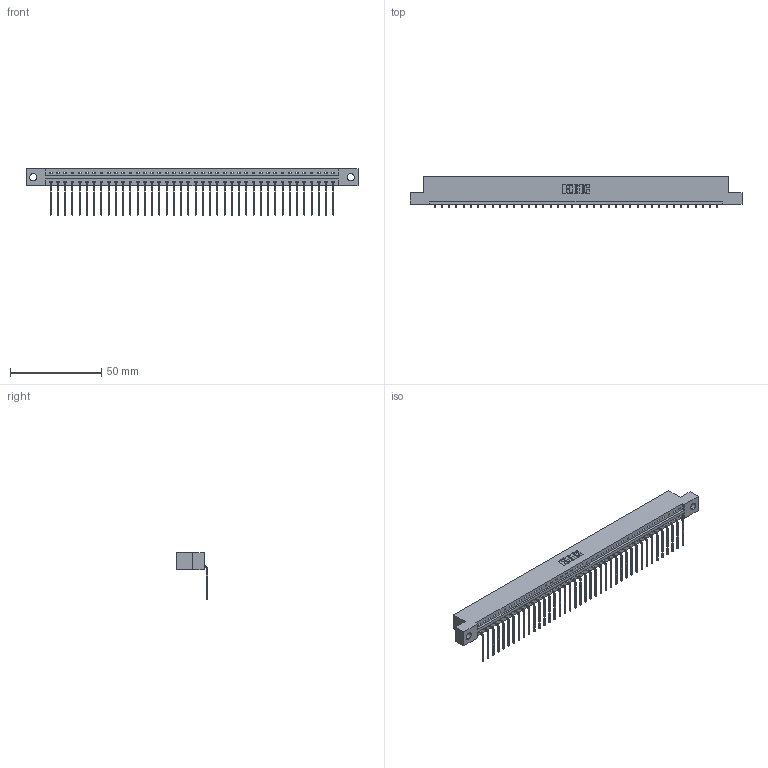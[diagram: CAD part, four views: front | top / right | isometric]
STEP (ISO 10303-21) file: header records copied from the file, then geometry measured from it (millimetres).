
FILE_DESCRIPTION (( 'STEP AP203' ), '1' );
FILE_NAME ('387-040-559-104.STEP', '2018-09-19T17:17:56', ( '' ), ( '' ), 'SwSTEP 2.0', 'SolidWorks 2016', '' );
FILE_SCHEMA (( 'CONFIG_CONTROL_DESIGN' ));
Length unit declared in the file: inch
Products named in the file (3): 337 Part_Flush Mounting Lugs - 0.156 Dia-TH; 345-292-001_558 559 Tail - 1; 387-040-559-104
Assembly tree (41 placements, depth 2):
  387-040-559-104
    337 Part_Flush Mounting Lugs - 0.156 Dia-TH
    345-292-001_558 559 Tail - 1  x40
Bounding box: 181.51 x 17.09 x 25.53 mm (x, y, z)
Volume: 18885.1 mm3; surface area: 20117.9 mm2
Topology: 41 solids, 41 shells, 2674 faces, 8071 edges, 5326 vertices
Faces by surface type: plane 1990, cylinder 684
Entity records: 30079 total; most frequent: CARTESIAN_POINT 5246, ORIENTED_EDGE 5222, DIRECTION 4419, EDGE_CURVE 2611, VECTOR 2483, LINE 2483, VERTEX_POINT 1738, AXIS2_PLACEMENT_3D 968
